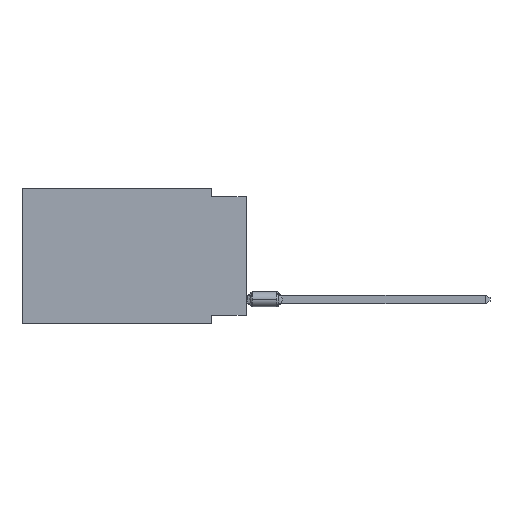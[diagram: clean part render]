
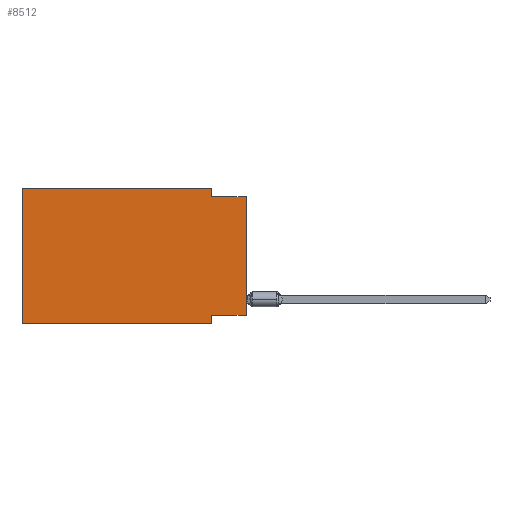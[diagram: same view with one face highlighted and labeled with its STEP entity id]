
A CAD part, left-side view. The second image highlights one B-rep face of the part: STEP entity #8512.
In plain terms, the highlighted planar face has unit normal (-1, 0, 0).
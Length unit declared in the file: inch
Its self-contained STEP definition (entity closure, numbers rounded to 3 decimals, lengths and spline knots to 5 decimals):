
#533 = LINE ( 'NONE', #7414, #3531 ) ;
#557 = CARTESIAN_POINT ( 'NONE',  ( 0., 0.645, 0. ) ) ;
#787 = DIRECTION ( 'NONE',  ( 0., 0., -1. ) ) ;
#811 = EDGE_CURVE ( 'NONE', #5569, #5811, #8005, .T. ) ;
#888 = ORIENTED_EDGE ( 'NONE', *, *, #8524, .F. ) ;
#956 = VERTEX_POINT ( 'NONE', #12584 ) ;
#1347 = CARTESIAN_POINT ( 'NONE',  ( 0., 0.645, -0.39 ) ) ;
#1467 = PLANE ( 'NONE',  #10168 ) ;
#1637 = CARTESIAN_POINT ( 'NONE',  ( 0., 0.645, 0. ) ) ;
#1723 = VECTOR ( 'NONE', #787, 39.37008 ) ;
#1912 = ORIENTED_EDGE ( 'NONE', *, *, #8903, .T. ) ;
#1963 = CARTESIAN_POINT ( 'NONE',  ( 0., 0.1, 0. ) ) ;
#2057 = CARTESIAN_POINT ( 'NONE',  ( 0., 0.1, -0.365 ) ) ;
#2381 = VECTOR ( 'NONE', #5747, 39.37008 ) ;
#2433 = DIRECTION ( 'NONE',  ( 0., 0., -1. ) ) ;
#2554 = CARTESIAN_POINT ( 'NONE',  ( 0., 0., -0.365 ) ) ;
#2654 = DIRECTION ( 'NONE',  ( 0., -1., 0. ) ) ;
#2738 = LINE ( 'NONE', #9675, #1723 ) ;
#3064 = CARTESIAN_POINT ( 'NONE',  ( 0., 0.645, -0.39 ) ) ;
#3216 = LINE ( 'NONE', #7441, #7898 ) ;
#3531 = VECTOR ( 'NONE', #6377, 39.37008 ) ;
#3661 = LINE ( 'NONE', #2554, #2381 ) ;
#4100 = CARTESIAN_POINT ( 'NONE',  ( 0., 0.645, 0. ) ) ;
#4897 = EDGE_CURVE ( 'NONE', #5912, #5811, #2738, .T. ) ;
#5438 = DIRECTION ( 'NONE',  ( 0., 0., -1. ) ) ;
#5529 = EDGE_LOOP ( 'NONE', ( #1912, #7246, #888, #11466, #8628, #6980, #10509, #10127 ) ) ;
#5569 = VERTEX_POINT ( 'NONE', #1347 ) ;
#5589 = LINE ( 'NONE', #5853, #6614 ) ;
#5609 = DIRECTION ( 'NONE',  ( 0., 0., 1. ) ) ;
#5666 = VERTEX_POINT ( 'NONE', #11132 ) ;
#5680 = CARTESIAN_POINT ( 'NONE',  ( 0., 0.645, 0. ) ) ;
#5747 = DIRECTION ( 'NONE',  ( 0., 1., 0. ) ) ;
#5811 = VERTEX_POINT ( 'NONE', #12617 ) ;
#5853 = CARTESIAN_POINT ( 'NONE',  ( 0., 0., -0.025 ) ) ;
#5912 = VERTEX_POINT ( 'NONE', #2057 ) ;
#6055 = LINE ( 'NONE', #4100, #7963 ) ;
#6178 = VERTEX_POINT ( 'NONE', #1963 ) ;
#6377 = DIRECTION ( 'NONE',  ( 0., 0., 1. ) ) ;
#6558 = EDGE_CURVE ( 'NONE', #956, #12602, #5589, .T. ) ;
#6614 = VECTOR ( 'NONE', #2654, 39.37008 ) ;
#6980 = ORIENTED_EDGE ( 'NONE', *, *, #811, .T. ) ;
#7040 = DIRECTION ( 'NONE',  ( 0., -1., 0. ) ) ;
#7246 = ORIENTED_EDGE ( 'NONE', *, *, #6558, .F. ) ;
#7414 = CARTESIAN_POINT ( 'NONE',  ( 0., 0., 0. ) ) ;
#7441 = CARTESIAN_POINT ( 'NONE',  ( 0., 0.1, 0. ) ) ;
#7680 = VECTOR ( 'NONE', #5609, 39.37008 ) ;
#7811 = EDGE_CURVE ( 'NONE', #5569, #7924, #9421, .T. ) ;
#7898 = VECTOR ( 'NONE', #5438, 39.37008 ) ;
#7924 = VERTEX_POINT ( 'NONE', #5680 ) ;
#7963 = VECTOR ( 'NONE', #8770, 39.37008 ) ;
#8005 = LINE ( 'NONE', #3064, #12793 ) ;
#8188 = CARTESIAN_POINT ( 'NONE',  ( 0., 0., -0.025 ) ) ;
#8465 = FACE_OUTER_BOUND ( 'NONE', #5529, .T. ) ;
#8512 = ADVANCED_FACE ( 'NONE', ( #8465 ), #1467, .F. ) ;
#8524 = EDGE_CURVE ( 'NONE', #6178, #956, #3216, .T. ) ;
#8628 = ORIENTED_EDGE ( 'NONE', *, *, #7811, .F. ) ;
#8770 = DIRECTION ( 'NONE',  ( 0., -1., 0. ) ) ;
#8903 = EDGE_CURVE ( 'NONE', #5666, #12602, #533, .T. ) ;
#9421 = LINE ( 'NONE', #1637, #7680 ) ;
#9675 = CARTESIAN_POINT ( 'NONE',  ( 0., 0.1, -0.39 ) ) ;
#10127 = ORIENTED_EDGE ( 'NONE', *, *, #10242, .F. ) ;
#10168 = AXIS2_PLACEMENT_3D ( 'NONE', #557, #10419, #2433 ) ;
#10242 = EDGE_CURVE ( 'NONE', #5666, #5912, #3661, .T. ) ;
#10419 = DIRECTION ( 'NONE',  ( 1., 0., 0. ) ) ;
#10509 = ORIENTED_EDGE ( 'NONE', *, *, #4897, .F. ) ;
#11132 = CARTESIAN_POINT ( 'NONE',  ( 0., 0., -0.365 ) ) ;
#11466 = ORIENTED_EDGE ( 'NONE', *, *, #12005, .F. ) ;
#12005 = EDGE_CURVE ( 'NONE', #7924, #6178, #6055, .T. ) ;
#12584 = CARTESIAN_POINT ( 'NONE',  ( 0., 0.1, -0.025 ) ) ;
#12602 = VERTEX_POINT ( 'NONE', #8188 ) ;
#12617 = CARTESIAN_POINT ( 'NONE',  ( 0., 0.1, -0.39 ) ) ;
#12793 = VECTOR ( 'NONE', #7040, 39.37008 ) ;
